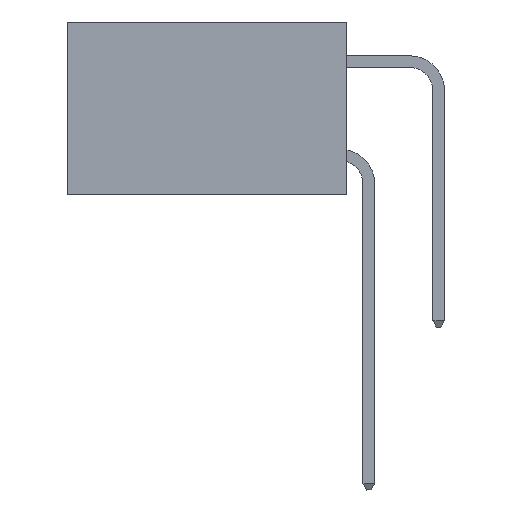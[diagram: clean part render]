
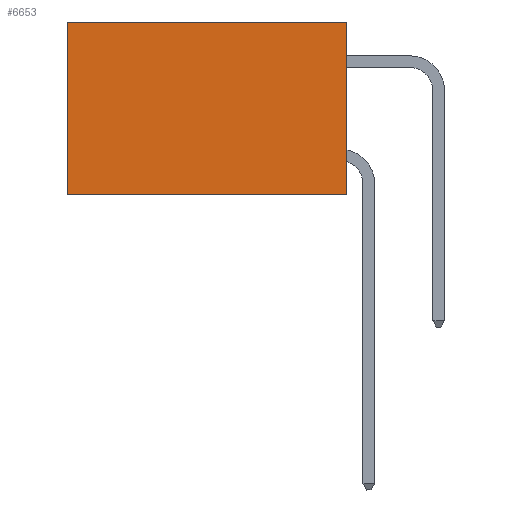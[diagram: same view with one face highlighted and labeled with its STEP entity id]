
A CAD part, left-side view. The second image highlights one B-rep face of the part: STEP entity #6653.
In plain terms, the highlighted planar face has unit normal (-1, 0, 0).
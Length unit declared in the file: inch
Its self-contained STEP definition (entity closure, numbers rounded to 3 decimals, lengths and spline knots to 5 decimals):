
#614 = ORIENTED_EDGE ( 'NONE', *, *, #20359, .F. ) ;
#726 = VERTEX_POINT ( 'NONE', #18692 ) ;
#1122 = DIRECTION ( 'NONE',  ( 0., 0., -1. ) ) ;
#1129 = DIRECTION ( 'NONE',  ( 1., 0., 0. ) ) ;
#1334 = PLANE ( 'NONE',  #11384 ) ;
#1677 = DIRECTION ( 'NONE',  ( 0., 1., 0. ) ) ;
#1730 = CARTESIAN_POINT ( 'NONE',  ( 0.2875, 0., 0. ) ) ;
#1773 = EDGE_CURVE ( 'NONE', #5939, #24151, #10444, .T. ) ;
#2492 = LINE ( 'NONE', #25419, #26744 ) ;
#4074 = DIRECTION ( 'NONE',  ( 0., 0., -1. ) ) ;
#4325 = CARTESIAN_POINT ( 'NONE',  ( 0.2875, 0., -0.37 ) ) ;
#4554 = CARTESIAN_POINT ( 'NONE',  ( 0.2875, 0.6, -0.37 ) ) ;
#4858 = CARTESIAN_POINT ( 'NONE',  ( 0.2875, 0., 0. ) ) ;
#5939 = VERTEX_POINT ( 'NONE', #4325 ) ;
#6653 = ADVANCED_FACE ( 'NONE', ( #20017 ), #1334, .F. ) ;
#7153 = LINE ( 'NONE', #18254, #21180 ) ;
#7219 = DIRECTION ( 'NONE',  ( 0., 1., 0. ) ) ;
#7942 = VECTOR ( 'NONE', #7219, 39.37008 ) ;
#8208 = VECTOR ( 'NONE', #1677, 39.37008 ) ;
#10444 = LINE ( 'NONE', #26034, #8208 ) ;
#10660 = ORIENTED_EDGE ( 'NONE', *, *, #23359, .T. ) ;
#11356 = EDGE_CURVE ( 'NONE', #726, #18845, #20499, .T. ) ;
#11384 = AXIS2_PLACEMENT_3D ( 'NONE', #1730, #1129, #1122 ) ;
#18254 = CARTESIAN_POINT ( 'NONE',  ( 0.2875, 0.6, 0. ) ) ;
#18692 = CARTESIAN_POINT ( 'NONE',  ( 0.2875, 0., 0. ) ) ;
#18845 = VERTEX_POINT ( 'NONE', #20322 ) ;
#19316 = ORIENTED_EDGE ( 'NONE', *, *, #1773, .F. ) ;
#20017 = FACE_OUTER_BOUND ( 'NONE', #26414, .T. ) ;
#20322 = CARTESIAN_POINT ( 'NONE',  ( 0.2875, 0.6, 0. ) ) ;
#20359 = EDGE_CURVE ( 'NONE', #726, #5939, #2492, .T. ) ;
#20499 = LINE ( 'NONE', #4858, #7942 ) ;
#21180 = VECTOR ( 'NONE', #4074, 39.37008 ) ;
#23359 = EDGE_CURVE ( 'NONE', #18845, #24151, #7153, .T. ) ;
#24151 = VERTEX_POINT ( 'NONE', #4554 ) ;
#25419 = CARTESIAN_POINT ( 'NONE',  ( 0.2875, 0., 0. ) ) ;
#26034 = CARTESIAN_POINT ( 'NONE',  ( 0.2875, 0., -0.37 ) ) ;
#26236 = ORIENTED_EDGE ( 'NONE', *, *, #11356, .T. ) ;
#26414 = EDGE_LOOP ( 'NONE', ( #10660, #19316, #614, #26236 ) ) ;
#26744 = VECTOR ( 'NONE', #27740, 39.37008 ) ;
#27740 = DIRECTION ( 'NONE',  ( 0., 0., -1. ) ) ;
